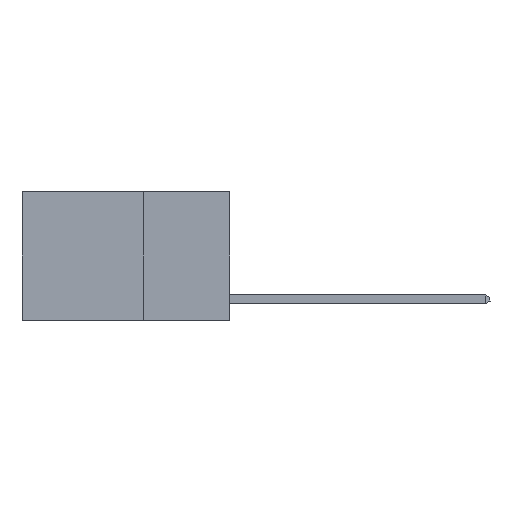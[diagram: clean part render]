
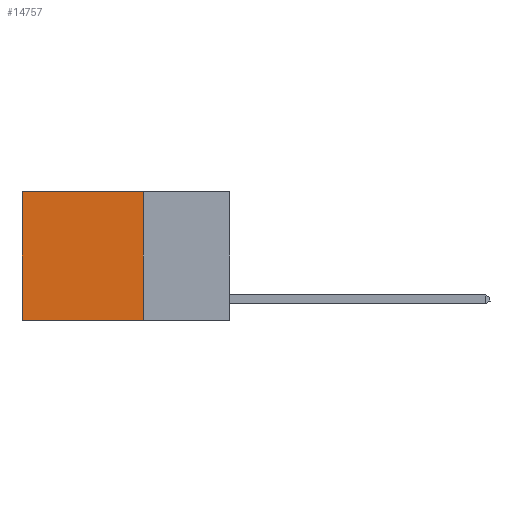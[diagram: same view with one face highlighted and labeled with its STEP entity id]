
A CAD part, left-side view. The second image highlights one B-rep face of the part: STEP entity #14757.
In plain terms, the highlighted planar face has unit normal (-1, 0, 0).
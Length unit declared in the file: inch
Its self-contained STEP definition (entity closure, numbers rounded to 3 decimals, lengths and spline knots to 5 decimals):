
#350 = DIRECTION ( 'NONE',  ( 0., 1., 0. ) ) ;
#647 = VECTOR ( 'NONE', #8695, 39.37008 ) ;
#979 = EDGE_CURVE ( 'NONE', #10144, #11340, #5968, .T. ) ;
#986 = ORIENTED_EDGE ( 'NONE', *, *, #15026, .F. ) ;
#1552 = VECTOR ( 'NONE', #10234, 39.37008 ) ;
#2056 = ORIENTED_EDGE ( 'NONE', *, *, #979, .T. ) ;
#3196 = CARTESIAN_POINT ( 'NONE',  ( 0.2625, 0.25, -0.37 ) ) ;
#4846 = LINE ( 'NONE', #6010, #8595 ) ;
#4903 = ORIENTED_EDGE ( 'NONE', *, *, #9207, .F. ) ;
#5350 = LINE ( 'NONE', #12993, #1552 ) ;
#5968 = LINE ( 'NONE', #12204, #9476 ) ;
#6010 = CARTESIAN_POINT ( 'NONE',  ( 0.2625, 0.25, -0.37 ) ) ;
#7080 = LINE ( 'NONE', #15750, #647 ) ;
#7281 = CARTESIAN_POINT ( 'NONE',  ( 0.2625, 0.25, 0. ) ) ;
#8292 = PLANE ( 'NONE',  #17567 ) ;
#8360 = CARTESIAN_POINT ( 'NONE',  ( 0.2625, 0.25, 0. ) ) ;
#8431 = DIRECTION ( 'NONE',  ( 0., 0., -1. ) ) ;
#8595 = VECTOR ( 'NONE', #350, 39.37008 ) ;
#8695 = DIRECTION ( 'NONE',  ( 0., 1., 0. ) ) ;
#9207 = EDGE_CURVE ( 'NONE', #18186, #16554, #5350, .T. ) ;
#9476 = VECTOR ( 'NONE', #17648, 39.37008 ) ;
#9717 = DIRECTION ( 'NONE',  ( 1., 0., 0. ) ) ;
#9985 = CARTESIAN_POINT ( 'NONE',  ( 0.2625, 0.6, -0.37 ) ) ;
#10144 = VERTEX_POINT ( 'NONE', #16122 ) ;
#10234 = DIRECTION ( 'NONE',  ( 0., 0., -1. ) ) ;
#11231 = FACE_OUTER_BOUND ( 'NONE', #13077, .T. ) ;
#11340 = VERTEX_POINT ( 'NONE', #9985 ) ;
#12204 = CARTESIAN_POINT ( 'NONE',  ( 0.2625, 0.6, 0. ) ) ;
#12993 = CARTESIAN_POINT ( 'NONE',  ( 0.2625, 0.25, 0. ) ) ;
#13077 = EDGE_LOOP ( 'NONE', ( #2056, #986, #4903, #15353 ) ) ;
#13491 = EDGE_CURVE ( 'NONE', #18186, #10144, #7080, .T. ) ;
#14757 = ADVANCED_FACE ( 'NONE', ( #11231 ), #8292, .F. ) ;
#15026 = EDGE_CURVE ( 'NONE', #16554, #11340, #4846, .T. ) ;
#15353 = ORIENTED_EDGE ( 'NONE', *, *, #13491, .T. ) ;
#15750 = CARTESIAN_POINT ( 'NONE',  ( 0.2625, 0.25, 0. ) ) ;
#16122 = CARTESIAN_POINT ( 'NONE',  ( 0.2625, 0.6, 0. ) ) ;
#16554 = VERTEX_POINT ( 'NONE', #3196 ) ;
#17567 = AXIS2_PLACEMENT_3D ( 'NONE', #8360, #9717, #8431 ) ;
#17648 = DIRECTION ( 'NONE',  ( 0., 0., -1. ) ) ;
#18186 = VERTEX_POINT ( 'NONE', #7281 ) ;
